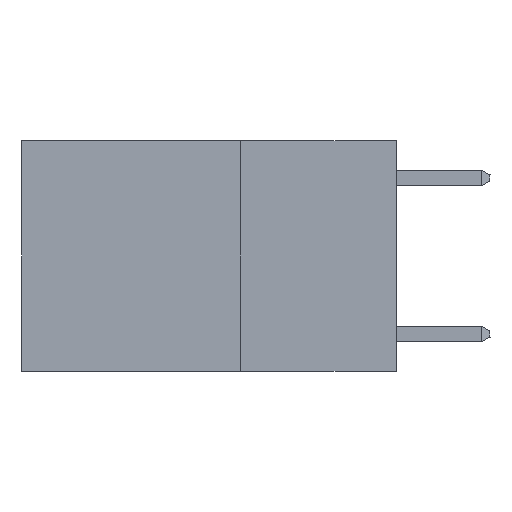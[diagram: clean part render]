
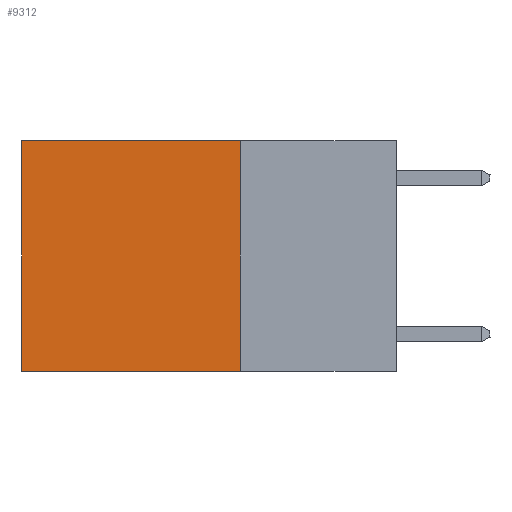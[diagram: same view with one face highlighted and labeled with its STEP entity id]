
A CAD part, left-side view. The second image highlights one B-rep face of the part: STEP entity #9312.
In plain terms, the highlighted planar face has unit normal (-1, 0, 0).
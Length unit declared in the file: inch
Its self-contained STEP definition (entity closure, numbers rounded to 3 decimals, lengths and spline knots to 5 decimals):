
#178 = VECTOR ( 'NONE', #935, 39.37008 ) ;
#621 = CARTESIAN_POINT ( 'NONE',  ( 0.2625, 0.6, 0. ) ) ;
#671 = DIRECTION ( 'NONE',  ( 0., 0., -1. ) ) ;
#715 = CARTESIAN_POINT ( 'NONE',  ( 0.2625, 0.25, 0. ) ) ;
#726 = CARTESIAN_POINT ( 'NONE',  ( 0.2625, 0.25, 0. ) ) ;
#935 = DIRECTION ( 'NONE',  ( 0., 1., 0. ) ) ;
#1307 = EDGE_CURVE ( 'NONE', #8412, #4586, #10463, .T. ) ;
#1641 = ORIENTED_EDGE ( 'NONE', *, *, #3043, .T. ) ;
#1790 = CARTESIAN_POINT ( 'NONE',  ( 0.2625, 0.25, 0. ) ) ;
#2174 = ORIENTED_EDGE ( 'NONE', *, *, #4202, .F. ) ;
#2355 = PLANE ( 'NONE',  #5986 ) ;
#2448 = VERTEX_POINT ( 'NONE', #8420 ) ;
#3043 = EDGE_CURVE ( 'NONE', #4586, #4988, #11221, .T. ) ;
#3990 = EDGE_CURVE ( 'NONE', #8412, #2448, #9565, .T. ) ;
#4202 = EDGE_CURVE ( 'NONE', #2448, #4988, #8838, .T. ) ;
#4352 = CARTESIAN_POINT ( 'NONE',  ( 0.2625, 0.25, 0. ) ) ;
#4586 = VERTEX_POINT ( 'NONE', #5314 ) ;
#4988 = VERTEX_POINT ( 'NONE', #8221 ) ;
#5086 = DIRECTION ( 'NONE',  ( 0., 0., -1. ) ) ;
#5314 = CARTESIAN_POINT ( 'NONE',  ( 0.2625, 0.6, 0. ) ) ;
#5986 = AXIS2_PLACEMENT_3D ( 'NONE', #726, #6843, #671 ) ;
#6835 = ORIENTED_EDGE ( 'NONE', *, *, #3990, .F. ) ;
#6843 = DIRECTION ( 'NONE',  ( 1., 0., 0. ) ) ;
#7042 = CARTESIAN_POINT ( 'NONE',  ( 0.2625, 0.25, -0.37 ) ) ;
#7192 = VECTOR ( 'NONE', #7854, 39.37008 ) ;
#7854 = DIRECTION ( 'NONE',  ( 0., 0., -1. ) ) ;
#8221 = CARTESIAN_POINT ( 'NONE',  ( 0.2625, 0.6, -0.37 ) ) ;
#8412 = VERTEX_POINT ( 'NONE', #715 ) ;
#8420 = CARTESIAN_POINT ( 'NONE',  ( 0.2625, 0.25, -0.37 ) ) ;
#8838 = LINE ( 'NONE', #7042, #178 ) ;
#8959 = ORIENTED_EDGE ( 'NONE', *, *, #1307, .T. ) ;
#9312 = ADVANCED_FACE ( 'NONE', ( #10284 ), #2355, .F. ) ;
#9565 = LINE ( 'NONE', #4352, #7192 ) ;
#9599 = DIRECTION ( 'NONE',  ( 0., 1., 0. ) ) ;
#9644 = VECTOR ( 'NONE', #5086, 39.37008 ) ;
#9816 = EDGE_LOOP ( 'NONE', ( #1641, #2174, #6835, #8959 ) ) ;
#10284 = FACE_OUTER_BOUND ( 'NONE', #9816, .T. ) ;
#10463 = LINE ( 'NONE', #1790, #11057 ) ;
#11057 = VECTOR ( 'NONE', #9599, 39.37008 ) ;
#11221 = LINE ( 'NONE', #621, #9644 ) ;
